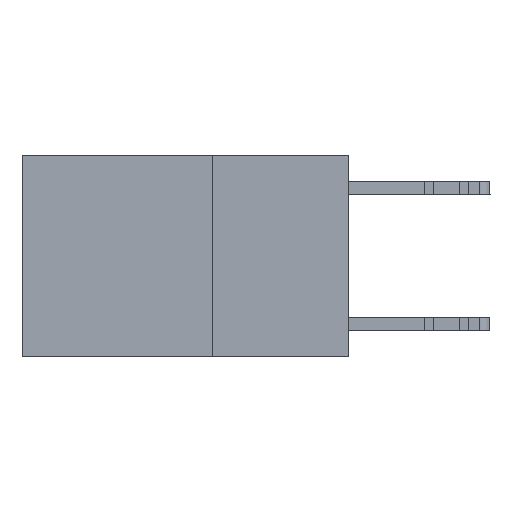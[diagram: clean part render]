
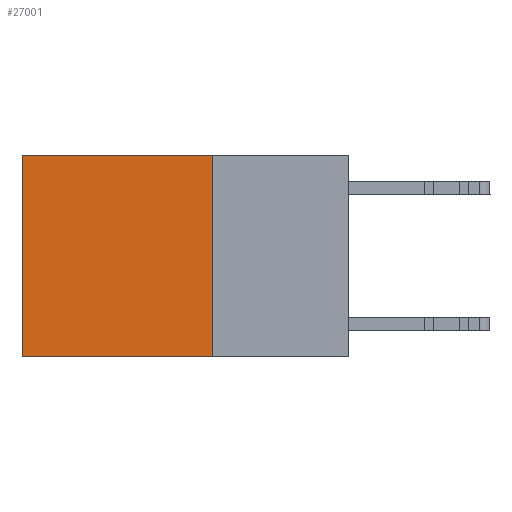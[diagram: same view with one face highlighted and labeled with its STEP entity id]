
A CAD part, left-side view. The second image highlights one B-rep face of the part: STEP entity #27001.
In plain terms, the highlighted planar face has unit normal (-1, 0, 0).
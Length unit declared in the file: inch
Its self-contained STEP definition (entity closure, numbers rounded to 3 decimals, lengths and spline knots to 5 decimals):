
#483 = AXIS2_PLACEMENT_3D ( 'NONE', #5842, #8099, #23569 ) ;
#902 = EDGE_LOOP ( 'NONE', ( #23768, #12559, #11040, #5212 ) ) ;
#1123 = CARTESIAN_POINT ( 'NONE',  ( 0.2625, 0.6, 0. ) ) ;
#1362 = VERTEX_POINT ( 'NONE', #25987 ) ;
#3672 = PLANE ( 'NONE',  #483 ) ;
#5212 = ORIENTED_EDGE ( 'NONE', *, *, #17256, .T. ) ;
#5842 = CARTESIAN_POINT ( 'NONE',  ( 0.2625, 0.25, 0. ) ) ;
#6617 = DIRECTION ( 'NONE',  ( 0., 1., 0. ) ) ;
#6962 = CARTESIAN_POINT ( 'NONE',  ( 0.2625, 0.25, 0. ) ) ;
#7717 = EDGE_CURVE ( 'NONE', #19630, #1362, #8972, .T. ) ;
#8099 = DIRECTION ( 'NONE',  ( 1., 0., 0. ) ) ;
#8949 = VECTOR ( 'NONE', #18462, 39.37008 ) ;
#8972 = LINE ( 'NONE', #1123, #8949 ) ;
#9350 = VERTEX_POINT ( 'NONE', #24069 ) ;
#11040 = ORIENTED_EDGE ( 'NONE', *, *, #17911, .F. ) ;
#12559 = ORIENTED_EDGE ( 'NONE', *, *, #24932, .F. ) ;
#12991 = CARTESIAN_POINT ( 'NONE',  ( 0.2625, 0.25, -0.37 ) ) ;
#14260 = DIRECTION ( 'NONE',  ( 0., 1., 0. ) ) ;
#14824 = CARTESIAN_POINT ( 'NONE',  ( 0.2625, 0.25, -0.37 ) ) ;
#16539 = VECTOR ( 'NONE', #14260, 39.37008 ) ;
#16672 = LINE ( 'NONE', #14824, #16539 ) ;
#17256 = EDGE_CURVE ( 'NONE', #9350, #19630, #27893, .T. ) ;
#17794 = FACE_OUTER_BOUND ( 'NONE', #902, .T. ) ;
#17911 = EDGE_CURVE ( 'NONE', #9350, #18587, #20402, .T. ) ;
#18462 = DIRECTION ( 'NONE',  ( 0., 0., -1. ) ) ;
#18587 = VERTEX_POINT ( 'NONE', #12991 ) ;
#19630 = VERTEX_POINT ( 'NONE', #25791 ) ;
#20235 = VECTOR ( 'NONE', #22134, 39.37008 ) ;
#20402 = LINE ( 'NONE', #22107, #20235 ) ;
#22107 = CARTESIAN_POINT ( 'NONE',  ( 0.2625, 0.25, 0. ) ) ;
#22134 = DIRECTION ( 'NONE',  ( 0., 0., -1. ) ) ;
#23569 = DIRECTION ( 'NONE',  ( 0., 0., -1. ) ) ;
#23768 = ORIENTED_EDGE ( 'NONE', *, *, #7717, .T. ) ;
#24069 = CARTESIAN_POINT ( 'NONE',  ( 0.2625, 0.25, 0. ) ) ;
#24932 = EDGE_CURVE ( 'NONE', #18587, #1362, #16672, .T. ) ;
#25791 = CARTESIAN_POINT ( 'NONE',  ( 0.2625, 0.6, 0. ) ) ;
#25987 = CARTESIAN_POINT ( 'NONE',  ( 0.2625, 0.6, -0.37 ) ) ;
#27001 = ADVANCED_FACE ( 'NONE', ( #17794 ), #3672, .F. ) ;
#27561 = VECTOR ( 'NONE', #6617, 39.37008 ) ;
#27893 = LINE ( 'NONE', #6962, #27561 ) ;
